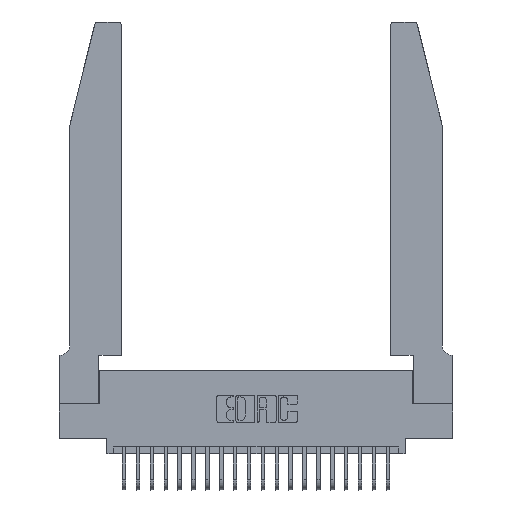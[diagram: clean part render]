
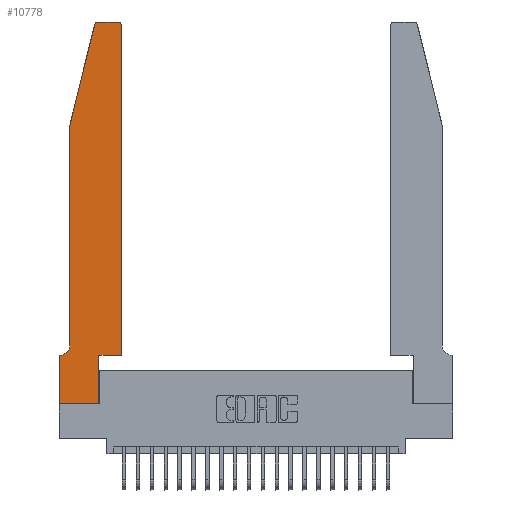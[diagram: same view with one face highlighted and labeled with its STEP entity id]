
A CAD part, top view. The second image highlights one B-rep face of the part: STEP entity #10778.
In plain terms, the highlighted planar face has unit normal (0, 0, 1).
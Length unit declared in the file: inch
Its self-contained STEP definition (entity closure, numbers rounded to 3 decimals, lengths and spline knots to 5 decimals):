
#1 = ORIENTED_EDGE ( 'NONE', *, *, #14812, .T. ) ;
#34 = DIRECTION ( 'NONE',  ( 1., 0., 0. ) ) ;
#150 = DIRECTION ( 'NONE',  ( -1., 0., 0. ) ) ;
#358 = VERTEX_POINT ( 'NONE', #7543 ) ;
#1816 = CARTESIAN_POINT ( 'NONE',  ( 0.4205, 2.72, 0.37 ) ) ;
#1928 = DIRECTION ( 'NONE',  ( 0., 0., 1. ) ) ;
#2058 = CARTESIAN_POINT ( 'NONE',  ( 0.0755, 0.35, 0.37 ) ) ;
#2409 = CIRCLE ( 'NONE', #6650, 0.03 ) ;
#2527 = DIRECTION ( 'NONE',  ( -0.239, -0.971, 0. ) ) ;
#2539 = LINE ( 'NONE', #2811, #16800 ) ;
#2573 = DIRECTION ( 'NONE',  ( -1., 0., 0. ) ) ;
#2811 = CARTESIAN_POINT ( 'NONE',  ( 0.2605, 2.75, 0.37 ) ) ;
#3133 = CARTESIAN_POINT ( 'NONE',  ( 0.0055, 0.35, 0.37 ) ) ;
#3312 = FACE_OUTER_BOUND ( 'NONE', #7740, .T. ) ;
#3417 = VECTOR ( 'NONE', #20602, 39.37008 ) ;
#3428 = ORIENTED_EDGE ( 'NONE', *, *, #24464, .T. ) ;
#3526 = CARTESIAN_POINT ( 'NONE',  ( 0.0755, 2., 0.37 ) ) ;
#3757 = DIRECTION ( 'NONE',  ( 0., 0., -1. ) ) ;
#4047 = EDGE_CURVE ( 'NONE', #7874, #11442, #6148, .T. ) ;
#4249 = VERTEX_POINT ( 'NONE', #3526 ) ;
#4709 = LINE ( 'NONE', #22415, #25162 ) ;
#5149 = DIRECTION ( 'NONE',  ( 0., -1., 0. ) ) ;
#5293 = ORIENTED_EDGE ( 'NONE', *, *, #5305, .T. ) ;
#5300 = CARTESIAN_POINT ( 'NONE',  ( 0.2865, 0.35, 0.37 ) ) ;
#5305 = EDGE_CURVE ( 'NONE', #18204, #21076, #15508, .T. ) ;
#5374 = AXIS2_PLACEMENT_3D ( 'NONE', #11649, #1928, #34 ) ;
#5764 = VERTEX_POINT ( 'NONE', #12232 ) ;
#5904 = CARTESIAN_POINT ( 'NONE',  ( 0.4505, 0.35, 0.37 ) ) ;
#6148 = CIRCLE ( 'NONE', #6696, 0.03 ) ;
#6150 = LINE ( 'NONE', #14776, #15213 ) ;
#6196 = ORIENTED_EDGE ( 'NONE', *, *, #24056, .T. ) ;
#6260 = CARTESIAN_POINT ( 'NONE',  ( 0.0755, 2., 0.37 ) ) ;
#6650 = AXIS2_PLACEMENT_3D ( 'NONE', #1816, #20911, #11537 ) ;
#6696 = AXIS2_PLACEMENT_3D ( 'NONE', #18258, #22174, #10490 ) ;
#7308 = CARTESIAN_POINT ( 'NONE',  ( 0., 0., 0.37 ) ) ;
#7543 = CARTESIAN_POINT ( 'NONE',  ( 0.4205, 2.75, 0.37 ) ) ;
#7740 = EDGE_LOOP ( 'NONE', ( #21204, #10909, #7790, #9362, #5293, #6196, #3428, #13934, #15064, #18006, #1, #19979 ) ) ;
#7790 = ORIENTED_EDGE ( 'NONE', *, *, #15724, .T. ) ;
#7874 = VERTEX_POINT ( 'NONE', #21499 ) ;
#7954 = DIRECTION ( 'NONE',  ( 1., 0., 0. ) ) ;
#8852 = VECTOR ( 'NONE', #16515, 39.37008 ) ;
#8999 = EDGE_CURVE ( 'NONE', #14234, #21655, #22888, .T. ) ;
#9250 = CARTESIAN_POINT ( 'NONE',  ( 0.0055, 0.42, 0.37 ) ) ;
#9362 = ORIENTED_EDGE ( 'NONE', *, *, #24249, .T. ) ;
#9711 = CARTESIAN_POINT ( 'NONE',  ( 0., 0.35, 0.37 ) ) ;
#10221 = CARTESIAN_POINT ( 'NONE',  ( 0.2865, 0., 0.37 ) ) ;
#10241 = LINE ( 'NONE', #22218, #20021 ) ;
#10374 = VECTOR ( 'NONE', #150, 39.37008 ) ;
#10490 = DIRECTION ( 'NONE',  ( 1., 0., 0. ) ) ;
#10778 = ADVANCED_FACE ( 'NONE', ( #3312 ), #23368, .T. ) ;
#10829 = EDGE_CURVE ( 'NONE', #5764, #358, #2409, .T. ) ;
#10909 = ORIENTED_EDGE ( 'NONE', *, *, #4047, .T. ) ;
#11038 = VERTEX_POINT ( 'NONE', #24388 ) ;
#11442 = VERTEX_POINT ( 'NONE', #13253 ) ;
#11537 = DIRECTION ( 'NONE',  ( 1., 0., 0. ) ) ;
#11649 = CARTESIAN_POINT ( 'NONE',  ( 0., 0.35, 0.37 ) ) ;
#11858 = VERTEX_POINT ( 'NONE', #7308 ) ;
#12232 = CARTESIAN_POINT ( 'NONE',  ( 0.4505, 2.72, 0.37 ) ) ;
#13020 = DIRECTION ( 'NONE',  ( 0., 1., 0. ) ) ;
#13253 = CARTESIAN_POINT ( 'NONE',  ( 0.25487, 2.72718, 0.37 ) ) ;
#13934 = ORIENTED_EDGE ( 'NONE', *, *, #19758, .T. ) ;
#14105 = CARTESIAN_POINT ( 'NONE',  ( 0.0755, 2., 0.37 ) ) ;
#14234 = VERTEX_POINT ( 'NONE', #10221 ) ;
#14612 = LINE ( 'NONE', #6260, #8852 ) ;
#14776 = CARTESIAN_POINT ( 'NONE',  ( 0., 0., 0.37 ) ) ;
#14812 = EDGE_CURVE ( 'NONE', #11038, #5764, #4709, .T. ) ;
#15064 = ORIENTED_EDGE ( 'NONE', *, *, #8999, .T. ) ;
#15213 = VECTOR ( 'NONE', #5149, 39.37008 ) ;
#15508 = CIRCLE ( 'NONE', #18770, 0.07 ) ;
#15724 = EDGE_CURVE ( 'NONE', #11442, #4249, #17128, .T. ) ;
#15918 = CARTESIAN_POINT ( 'NONE',  ( 0.0755, 0.42, 0.37 ) ) ;
#16515 = DIRECTION ( 'NONE',  ( 0., -1., 0. ) ) ;
#16800 = VECTOR ( 'NONE', #2573, 39.37008 ) ;
#16933 = VECTOR ( 'NONE', #7954, 39.37008 ) ;
#16946 = EDGE_CURVE ( 'NONE', #358, #7874, #2539, .T. ) ;
#17128 = LINE ( 'NONE', #14105, #24194 ) ;
#18006 = ORIENTED_EDGE ( 'NONE', *, *, #21397, .T. ) ;
#18204 = VERTEX_POINT ( 'NONE', #15918 ) ;
#18258 = CARTESIAN_POINT ( 'NONE',  ( 0.284, 2.72, 0.37 ) ) ;
#18770 = AXIS2_PLACEMENT_3D ( 'NONE', #9250, #3757, #22894 ) ;
#19241 = VERTEX_POINT ( 'NONE', #9711 ) ;
#19758 = EDGE_CURVE ( 'NONE', #11858, #14234, #10241, .T. ) ;
#19979 = ORIENTED_EDGE ( 'NONE', *, *, #10829, .T. ) ;
#20021 = VECTOR ( 'NONE', #24395, 39.37008 ) ;
#20436 = CARTESIAN_POINT ( 'NONE',  ( 0.2865, 0.35, 0.37 ) ) ;
#20602 = DIRECTION ( 'NONE',  ( 0., 1., 0. ) ) ;
#20761 = LINE ( 'NONE', #2058, #10374 ) ;
#20911 = DIRECTION ( 'NONE',  ( 0., 0., 1. ) ) ;
#21076 = VERTEX_POINT ( 'NONE', #3133 ) ;
#21204 = ORIENTED_EDGE ( 'NONE', *, *, #16946, .T. ) ;
#21397 = EDGE_CURVE ( 'NONE', #21655, #11038, #22108, .T. ) ;
#21499 = CARTESIAN_POINT ( 'NONE',  ( 0.284, 2.75, 0.37 ) ) ;
#21655 = VERTEX_POINT ( 'NONE', #5300 ) ;
#22108 = LINE ( 'NONE', #5904, #16933 ) ;
#22174 = DIRECTION ( 'NONE',  ( 0., 0., 1. ) ) ;
#22218 = CARTESIAN_POINT ( 'NONE',  ( 0., 0., 0.37 ) ) ;
#22415 = CARTESIAN_POINT ( 'NONE',  ( 0.4505, 0.35, 0.37 ) ) ;
#22888 = LINE ( 'NONE', #20436, #3417 ) ;
#22894 = DIRECTION ( 'NONE',  ( -1., 0., 0. ) ) ;
#23368 = PLANE ( 'NONE',  #5374 ) ;
#24056 = EDGE_CURVE ( 'NONE', #21076, #19241, #20761, .T. ) ;
#24194 = VECTOR ( 'NONE', #2527, 39.37008 ) ;
#24249 = EDGE_CURVE ( 'NONE', #4249, #18204, #14612, .T. ) ;
#24388 = CARTESIAN_POINT ( 'NONE',  ( 0.4505, 0.35, 0.37 ) ) ;
#24395 = DIRECTION ( 'NONE',  ( 1., 0., 0. ) ) ;
#24464 = EDGE_CURVE ( 'NONE', #19241, #11858, #6150, .T. ) ;
#25162 = VECTOR ( 'NONE', #13020, 39.37008 ) ;
